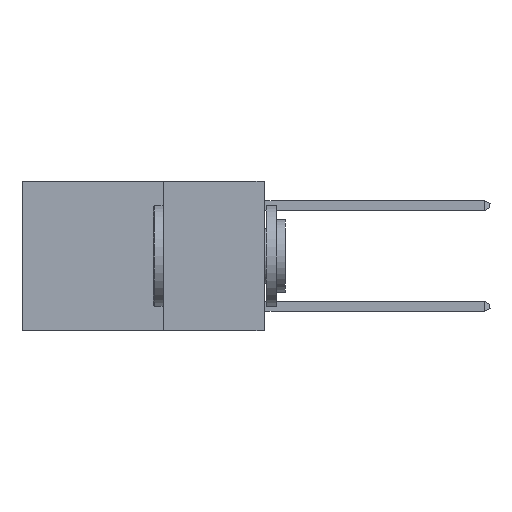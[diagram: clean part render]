
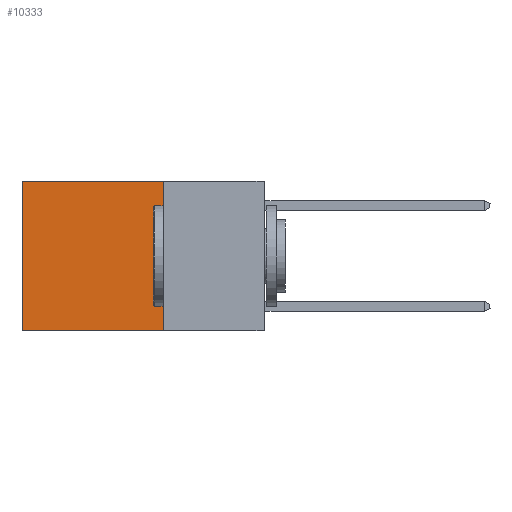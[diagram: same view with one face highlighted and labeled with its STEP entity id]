
A CAD part, left-side view. The second image highlights one B-rep face of the part: STEP entity #10333.
In plain terms, the highlighted planar face has unit normal (-1, 0, 0).
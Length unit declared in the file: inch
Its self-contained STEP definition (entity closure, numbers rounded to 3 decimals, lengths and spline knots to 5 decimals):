
#190 = EDGE_CURVE ( 'NONE', #9143, #4700, #1648, .T. ) ;
#903 = CARTESIAN_POINT ( 'NONE',  ( 0.2625, 0.25, -0.37 ) ) ;
#958 = EDGE_CURVE ( 'NONE', #2895, #3600, #7683, .T. ) ;
#988 = EDGE_CURVE ( 'NONE', #9143, #2895, #4905, .T. ) ;
#1082 = EDGE_LOOP ( 'NONE', ( #4551, #5166, #9796, #4125 ) ) ;
#1322 = EDGE_CURVE ( 'NONE', #4700, #3600, #8624, .T. ) ;
#1648 = LINE ( 'NONE', #3603, #8044 ) ;
#1813 = VECTOR ( 'NONE', #10350, 39.37008 ) ;
#2330 = DIRECTION ( 'NONE',  ( 0., 0., -1. ) ) ;
#2895 = VERTEX_POINT ( 'NONE', #903 ) ;
#2976 = DIRECTION ( 'NONE',  ( 1., 0., 0. ) ) ;
#3600 = VERTEX_POINT ( 'NONE', #6870 ) ;
#3603 = CARTESIAN_POINT ( 'NONE',  ( 0.2625, 0.25, 0. ) ) ;
#4125 = ORIENTED_EDGE ( 'NONE', *, *, #190, .T. ) ;
#4472 = DIRECTION ( 'NONE',  ( 0., 1., 0. ) ) ;
#4551 = ORIENTED_EDGE ( 'NONE', *, *, #1322, .T. ) ;
#4700 = VERTEX_POINT ( 'NONE', #7183 ) ;
#4905 = LINE ( 'NONE', #7557, #1813 ) ;
#5166 = ORIENTED_EDGE ( 'NONE', *, *, #958, .F. ) ;
#5629 = PLANE ( 'NONE',  #9090 ) ;
#6870 = CARTESIAN_POINT ( 'NONE',  ( 0.2625, 0.6, -0.37 ) ) ;
#7183 = CARTESIAN_POINT ( 'NONE',  ( 0.2625, 0.6, 0. ) ) ;
#7500 = DIRECTION ( 'NONE',  ( 0., 1., 0. ) ) ;
#7557 = CARTESIAN_POINT ( 'NONE',  ( 0.2625, 0.25, 0. ) ) ;
#7683 = LINE ( 'NONE', #11226, #9737 ) ;
#8044 = VECTOR ( 'NONE', #4472, 39.37008 ) ;
#8624 = LINE ( 'NONE', #8685, #9923 ) ;
#8685 = CARTESIAN_POINT ( 'NONE',  ( 0.2625, 0.6, 0. ) ) ;
#9090 = AXIS2_PLACEMENT_3D ( 'NONE', #10915, #2976, #9328 ) ;
#9143 = VERTEX_POINT ( 'NONE', #9213 ) ;
#9213 = CARTESIAN_POINT ( 'NONE',  ( 0.2625, 0.25, 0. ) ) ;
#9328 = DIRECTION ( 'NONE',  ( 0., 0., -1. ) ) ;
#9737 = VECTOR ( 'NONE', #7500, 39.37008 ) ;
#9796 = ORIENTED_EDGE ( 'NONE', *, *, #988, .F. ) ;
#9923 = VECTOR ( 'NONE', #2330, 39.37008 ) ;
#10333 = ADVANCED_FACE ( 'NONE', ( #11151 ), #5629, .F. ) ;
#10350 = DIRECTION ( 'NONE',  ( 0., 0., -1. ) ) ;
#10915 = CARTESIAN_POINT ( 'NONE',  ( 0.2625, 0.25, 0. ) ) ;
#11151 = FACE_OUTER_BOUND ( 'NONE', #1082, .T. ) ;
#11226 = CARTESIAN_POINT ( 'NONE',  ( 0.2625, 0.25, -0.37 ) ) ;
